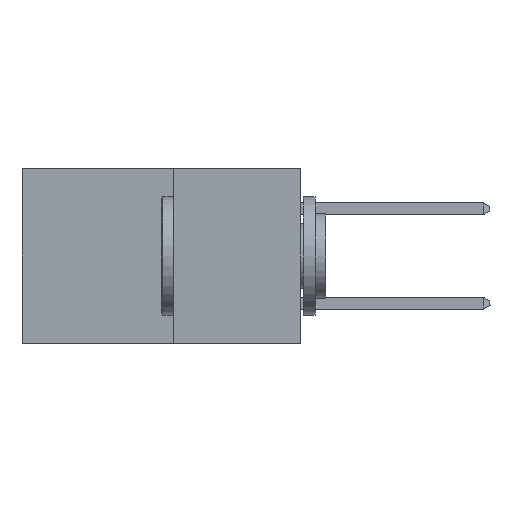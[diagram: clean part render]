
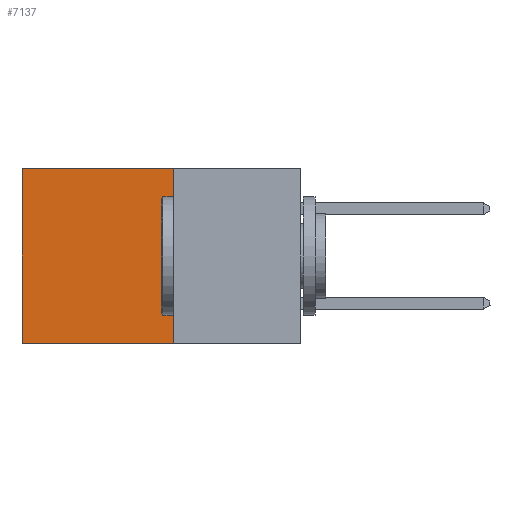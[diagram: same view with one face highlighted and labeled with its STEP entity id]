
A CAD part, left-side view. The second image highlights one B-rep face of the part: STEP entity #7137.
In plain terms, the highlighted planar face has unit normal (-1, 0, 0).
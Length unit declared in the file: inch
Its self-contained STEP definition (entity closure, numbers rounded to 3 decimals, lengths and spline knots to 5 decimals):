
#348 = DIRECTION ( 'NONE',  ( 0., 0., -1. ) ) ;
#436 = CARTESIAN_POINT ( 'NONE',  ( 0.277, 0.59, -0.37 ) ) ;
#988 = VERTEX_POINT ( 'NONE', #15171 ) ;
#1107 = EDGE_LOOP ( 'NONE', ( #2073, #17780, #16280, #1673 ) ) ;
#1673 = ORIENTED_EDGE ( 'NONE', *, *, #17737, .T. ) ;
#2073 = ORIENTED_EDGE ( 'NONE', *, *, #6825, .T. ) ;
#2903 = LINE ( 'NONE', #9017, #11415 ) ;
#3372 = VERTEX_POINT ( 'NONE', #15667 ) ;
#3601 = LINE ( 'NONE', #436, #19734 ) ;
#3863 = LINE ( 'NONE', #7945, #15975 ) ;
#5009 = AXIS2_PLACEMENT_3D ( 'NONE', #5485, #7117, #18061 ) ;
#5485 = CARTESIAN_POINT ( 'NONE',  ( 0.277, 0.27, -0.37 ) ) ;
#5611 = EDGE_CURVE ( 'NONE', #3372, #988, #2903, .T. ) ;
#5616 = VERTEX_POINT ( 'NONE', #8483 ) ;
#6825 = EDGE_CURVE ( 'NONE', #13016, #5616, #3601, .T. ) ;
#7117 = DIRECTION ( 'NONE',  ( 1., 0., 0. ) ) ;
#7137 = ADVANCED_FACE ( 'NONE', ( #15497 ), #16521, .F. ) ;
#7945 = CARTESIAN_POINT ( 'NONE',  ( 0.277, 0.27, 0. ) ) ;
#8483 = CARTESIAN_POINT ( 'NONE',  ( 0.277, 0.59, -0.37 ) ) ;
#8697 = DIRECTION ( 'NONE',  ( 0., 0., -1. ) ) ;
#8860 = VECTOR ( 'NONE', #11228, 39.37008 ) ;
#9017 = CARTESIAN_POINT ( 'NONE',  ( 0.277, 0.27, -0.37 ) ) ;
#11228 = DIRECTION ( 'NONE',  ( 0., 1., 0. ) ) ;
#11415 = VECTOR ( 'NONE', #8697, 39.37008 ) ;
#12446 = CARTESIAN_POINT ( 'NONE',  ( 0.277, 0.59, 0. ) ) ;
#13016 = VERTEX_POINT ( 'NONE', #12446 ) ;
#13039 = LINE ( 'NONE', #17358, #8860 ) ;
#14092 = EDGE_CURVE ( 'NONE', #988, #5616, #13039, .T. ) ;
#14252 = DIRECTION ( 'NONE',  ( 0., 1., 0. ) ) ;
#15171 = CARTESIAN_POINT ( 'NONE',  ( 0.277, 0.27, -0.37 ) ) ;
#15497 = FACE_OUTER_BOUND ( 'NONE', #1107, .T. ) ;
#15667 = CARTESIAN_POINT ( 'NONE',  ( 0.277, 0.27, 0. ) ) ;
#15975 = VECTOR ( 'NONE', #14252, 39.37008 ) ;
#16280 = ORIENTED_EDGE ( 'NONE', *, *, #5611, .F. ) ;
#16521 = PLANE ( 'NONE',  #5009 ) ;
#17358 = CARTESIAN_POINT ( 'NONE',  ( 0.277, 0.27, -0.37 ) ) ;
#17737 = EDGE_CURVE ( 'NONE', #3372, #13016, #3863, .T. ) ;
#17780 = ORIENTED_EDGE ( 'NONE', *, *, #14092, .F. ) ;
#18061 = DIRECTION ( 'NONE',  ( 0., 0., -1. ) ) ;
#19734 = VECTOR ( 'NONE', #348, 39.37008 ) ;
